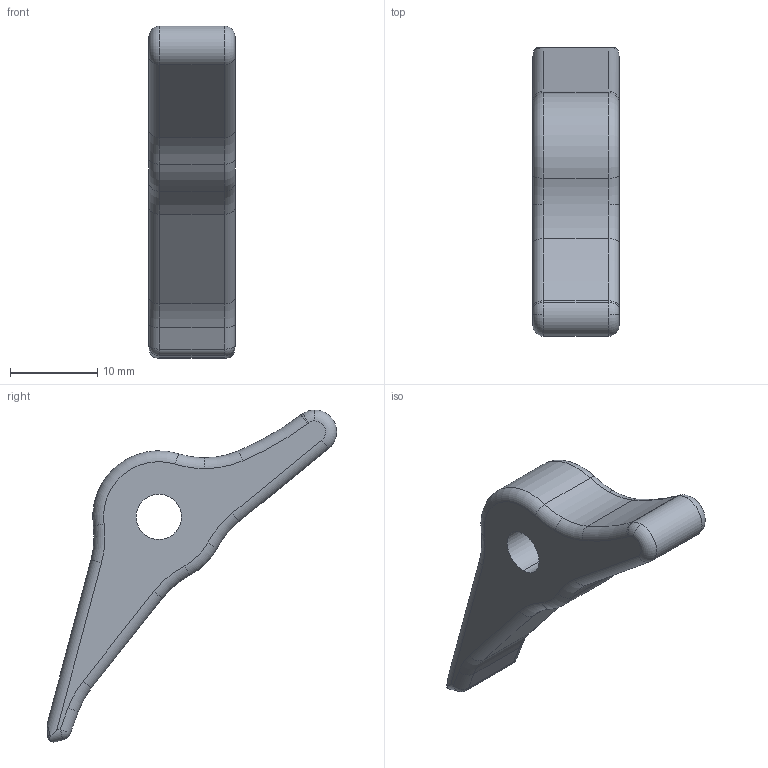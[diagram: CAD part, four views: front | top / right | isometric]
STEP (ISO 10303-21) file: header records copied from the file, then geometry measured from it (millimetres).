
FILE_DESCRIPTION (( 'STEP AP214' ), '1' );
FILE_NAME ('Trigger.STEP', '2014-02-20T01:03:42', ( '' ), ( '' ), 'SwSTEP 2.0', 'SolidWorks 2013', '' );
FILE_SCHEMA (( 'AUTOMOTIVE_DESIGN' ));
Length unit declared in the file: millimetre
Products named in the file (1): Trigger
Bounding box: 9.9 x 33.23 x 38.16 mm (x, y, z)
Volume: 3622.2 mm3; surface area: 1892.3 mm2
Topology: 1 solids, 1 shells, 66 faces, 156 edges, 90 vertices
Faces by surface type: cylinder 26, torus 24, plane 8, bspline 6, sphere 2
Entity records: 2014 total; most frequent: CARTESIAN_POINT 475, DIRECTION 348, ORIENTED_EDGE 308, EDGE_CURVE 154, AXIS2_PLACEMENT_3D 153, CIRCLE 92, VERTEX_POINT 90, EDGE_LOOP 68
